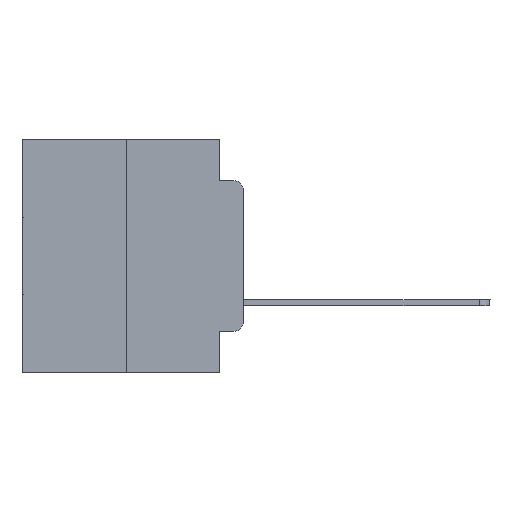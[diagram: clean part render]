
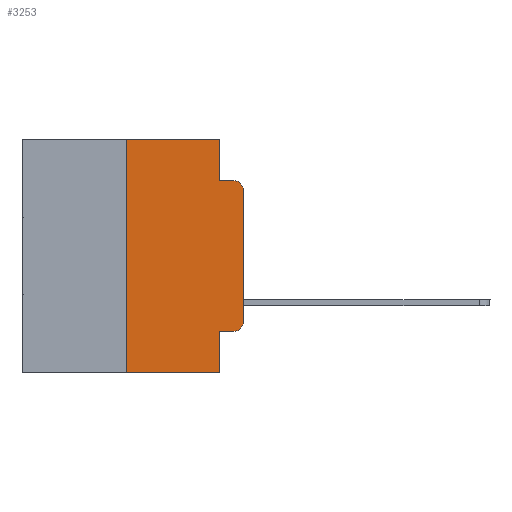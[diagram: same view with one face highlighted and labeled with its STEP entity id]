
A CAD part, left-side view. The second image highlights one B-rep face of the part: STEP entity #3253.
In plain terms, the highlighted planar face has unit normal (-1, 0, 0).
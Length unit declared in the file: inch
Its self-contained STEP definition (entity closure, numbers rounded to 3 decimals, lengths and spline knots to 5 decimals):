
#6 = ORIENTED_EDGE ( 'NONE', *, *, #20112, .F. ) ;
#450 = LINE ( 'NONE', #6764, #23018 ) ;
#733 = ORIENTED_EDGE ( 'NONE', *, *, #20712, .T. ) ;
#947 = DIRECTION ( 'NONE',  ( 0., 0., -1. ) ) ;
#1452 = CARTESIAN_POINT ( 'NONE',  ( 0., 0.02, -0.4115 ) ) ;
#2312 = LINE ( 'NONE', #12031, #3678 ) ;
#3140 = ORIENTED_EDGE ( 'NONE', *, *, #9863, .F. ) ;
#3196 = LINE ( 'NONE', #18752, #13431 ) ;
#3253 = ADVANCED_FACE ( 'NONE', ( #10551 ), #11229, .F. ) ;
#3678 = VECTOR ( 'NONE', #27325, 39.37008 ) ;
#3694 = VERTEX_POINT ( 'NONE', #10881 ) ;
#3788 = LINE ( 'NONE', #23891, #9945 ) ;
#3991 = EDGE_CURVE ( 'NONE', #3694, #18854, #2312, .T. ) ;
#4005 = ORIENTED_EDGE ( 'NONE', *, *, #8315, .T. ) ;
#4172 = LINE ( 'NONE', #25174, #19876 ) ;
#4417 = VERTEX_POINT ( 'NONE', #18574 ) ;
#4494 = VERTEX_POINT ( 'NONE', #7982 ) ;
#4917 = CARTESIAN_POINT ( 'NONE',  ( 0., 0.051, -0.5 ) ) ;
#5254 = AXIS2_PLACEMENT_3D ( 'NONE', #8859, #13239, #15452 ) ;
#5405 = CIRCLE ( 'NONE', #22251, 0.02 ) ;
#5447 = DIRECTION ( 'NONE',  ( 0., 0., -1. ) ) ;
#5589 = CARTESIAN_POINT ( 'NONE',  ( 0., 0.051, -0.0885 ) ) ;
#5739 = CARTESIAN_POINT ( 'NONE',  ( 0., 0.02, -0.0885 ) ) ;
#5931 = VECTOR ( 'NONE', #5447, 39.37008 ) ;
#6314 = EDGE_CURVE ( 'NONE', #22730, #16110, #11079, .T. ) ;
#6761 = DIRECTION ( 'NONE',  ( 0., 0., -1. ) ) ;
#6764 = CARTESIAN_POINT ( 'NONE',  ( 0., 0., 0. ) ) ;
#7152 = VERTEX_POINT ( 'NONE', #8579 ) ;
#7173 = ORIENTED_EDGE ( 'NONE', *, *, #7792, .F. ) ;
#7352 = DIRECTION ( 'NONE',  ( -1., 0., 0. ) ) ;
#7470 = DIRECTION ( 'NONE',  ( -1., 0., 0. ) ) ;
#7556 = DIRECTION ( 'NONE',  ( 0., 0., -1. ) ) ;
#7767 = ORIENTED_EDGE ( 'NONE', *, *, #10844, .T. ) ;
#7792 = EDGE_CURVE ( 'NONE', #3694, #11628, #11043, .T. ) ;
#7860 = DIRECTION ( 'NONE',  ( 0., -1., 0. ) ) ;
#7982 = CARTESIAN_POINT ( 'NONE',  ( 0., 0., -0.1085 ) ) ;
#8315 = EDGE_CURVE ( 'NONE', #21399, #11628, #4172, .T. ) ;
#8579 = CARTESIAN_POINT ( 'NONE',  ( 0., 0.051, 0. ) ) ;
#8859 = CARTESIAN_POINT ( 'NONE',  ( 0., 0.473, 0. ) ) ;
#9863 = EDGE_CURVE ( 'NONE', #4417, #7152, #10933, .T. ) ;
#9945 = VECTOR ( 'NONE', #6761, 39.37008 ) ;
#10152 = DIRECTION ( 'NONE',  ( 0., -1., 0. ) ) ;
#10551 = FACE_OUTER_BOUND ( 'NONE', #19918, .T. ) ;
#10672 = DIRECTION ( 'NONE',  ( 0., 0., 1. ) ) ;
#10844 = EDGE_CURVE ( 'NONE', #4494, #16110, #25264, .T. ) ;
#10881 = CARTESIAN_POINT ( 'NONE',  ( 0., 0.051, -0.4115 ) ) ;
#10933 = LINE ( 'NONE', #19392, #15055 ) ;
#11043 = LINE ( 'NONE', #16218, #5931 ) ;
#11079 = LINE ( 'NONE', #5589, #16190 ) ;
#11164 = ORIENTED_EDGE ( 'NONE', *, *, #3991, .T. ) ;
#11229 = PLANE ( 'NONE',  #5254 ) ;
#11297 = EDGE_CURVE ( 'NONE', #18854, #21694, #5405, .T. ) ;
#11438 = CARTESIAN_POINT ( 'NONE',  ( 0., 0.25, -0.5 ) ) ;
#11628 = VERTEX_POINT ( 'NONE', #4917 ) ;
#12031 = CARTESIAN_POINT ( 'NONE',  ( 0., 0.051, -0.4115 ) ) ;
#13239 = DIRECTION ( 'NONE',  ( 1., 0., 0. ) ) ;
#13431 = VECTOR ( 'NONE', #21827, 39.37008 ) ;
#14793 = CARTESIAN_POINT ( 'NONE',  ( 0., 0., -0.3915 ) ) ;
#15055 = VECTOR ( 'NONE', #19570, 39.37008 ) ;
#15452 = DIRECTION ( 'NONE',  ( 0., 0., -1. ) ) ;
#16017 = CARTESIAN_POINT ( 'NONE',  ( 0., 0.02, -0.1085 ) ) ;
#16110 = VERTEX_POINT ( 'NONE', #5739 ) ;
#16190 = VECTOR ( 'NONE', #10152, 39.37008 ) ;
#16218 = CARTESIAN_POINT ( 'NONE',  ( 0., 0.051, 0. ) ) ;
#17468 = ORIENTED_EDGE ( 'NONE', *, *, #11297, .T. ) ;
#17617 = ORIENTED_EDGE ( 'NONE', *, *, #21857, .F. ) ;
#18574 = CARTESIAN_POINT ( 'NONE',  ( 0., 0.25, 0. ) ) ;
#18752 = CARTESIAN_POINT ( 'NONE',  ( 0., 0.25, 0. ) ) ;
#18854 = VERTEX_POINT ( 'NONE', #1452 ) ;
#19392 = CARTESIAN_POINT ( 'NONE',  ( 0., 0.473, 0. ) ) ;
#19570 = DIRECTION ( 'NONE',  ( 0., -1., 0. ) ) ;
#19876 = VECTOR ( 'NONE', #7860, 39.37008 ) ;
#19918 = EDGE_LOOP ( 'NONE', ( #733, #7767, #20295, #17617, #3140, #6, #4005, #7173, #11164, #17468 ) ) ;
#20112 = EDGE_CURVE ( 'NONE', #21399, #4417, #3196, .T. ) ;
#20295 = ORIENTED_EDGE ( 'NONE', *, *, #6314, .F. ) ;
#20712 = EDGE_CURVE ( 'NONE', #21694, #4494, #450, .T. ) ;
#21399 = VERTEX_POINT ( 'NONE', #11438 ) ;
#21694 = VERTEX_POINT ( 'NONE', #14793 ) ;
#21827 = DIRECTION ( 'NONE',  ( 0., 0., 1. ) ) ;
#21857 = EDGE_CURVE ( 'NONE', #7152, #22730, #3788, .T. ) ;
#22251 = AXIS2_PLACEMENT_3D ( 'NONE', #27545, #7470, #947 ) ;
#22730 = VERTEX_POINT ( 'NONE', #22852 ) ;
#22794 = AXIS2_PLACEMENT_3D ( 'NONE', #16017, #7352, #7556 ) ;
#22852 = CARTESIAN_POINT ( 'NONE',  ( 0., 0.051, -0.0885 ) ) ;
#23018 = VECTOR ( 'NONE', #10672, 39.37008 ) ;
#23891 = CARTESIAN_POINT ( 'NONE',  ( 0., 0.051, 0. ) ) ;
#25174 = CARTESIAN_POINT ( 'NONE',  ( 0., 0.473, -0.5 ) ) ;
#25264 = CIRCLE ( 'NONE', #22794, 0.02 ) ;
#27325 = DIRECTION ( 'NONE',  ( 0., -1., 0. ) ) ;
#27545 = CARTESIAN_POINT ( 'NONE',  ( 0., 0.02, -0.3915 ) ) ;
